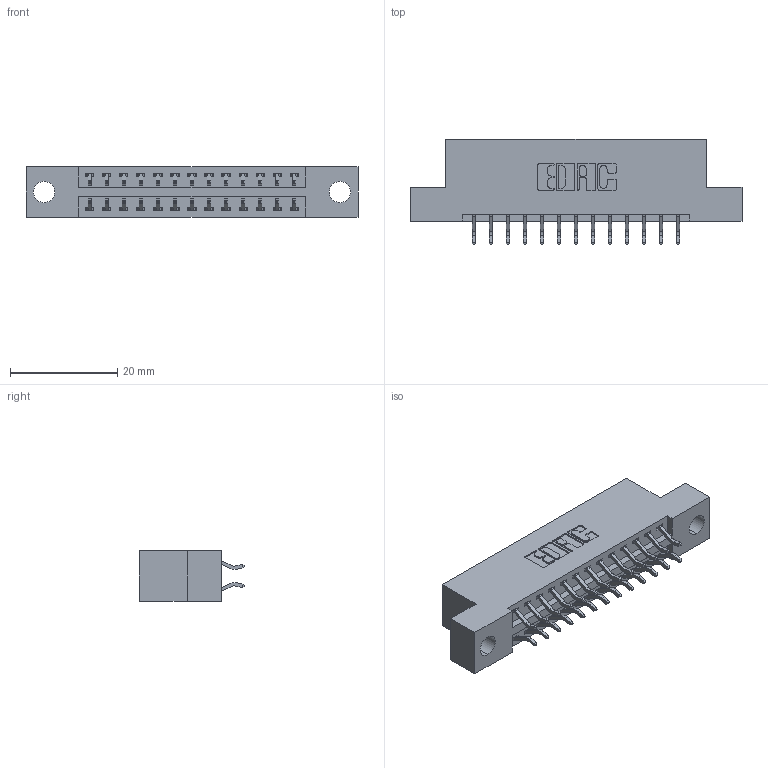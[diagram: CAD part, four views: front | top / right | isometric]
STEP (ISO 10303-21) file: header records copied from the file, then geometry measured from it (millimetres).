
FILE_DESCRIPTION (( 'STEP AP203' ), '1' );
FILE_NAME ('346-026-556-204.STEP', '2022-05-19T02:29:28', ( '' ), ( '' ), 'SwSTEP 2.0', 'SolidWorks 2020', '' );
FILE_SCHEMA (( 'CONFIG_CONTROL_DESIGN' ));
Length unit declared in the file: inch
Products named in the file (3): 346 Part_Flush Mounting Lugs - 0.156 Dia-TH; 345-292-001_556 Tail; 346-026-556-204
Assembly tree (27 placements, depth 2):
  346-026-556-204
    346 Part_Flush Mounting Lugs - 0.156 Dia-TH
    345-292-001_556 Tail  x26
Bounding box: 61.85 x 19.57 x 9.4 mm (x, y, z)
Volume: 5698.8 mm3; surface area: 7201.4 mm2
Topology: 27 solids, 27 shells, 1644 faces, 4863 edges, 3206 vertices
Faces by surface type: plane 1104, cylinder 540
Entity records: 13027 total; most frequent: CARTESIAN_POINT 2206, ORIENTED_EDGE 2126, DIRECTION 1983, EDGE_CURVE 1063, VECTOR 871, LINE 871, VERTEX_POINT 706, AXIS2_PLACEMENT_3D 556
